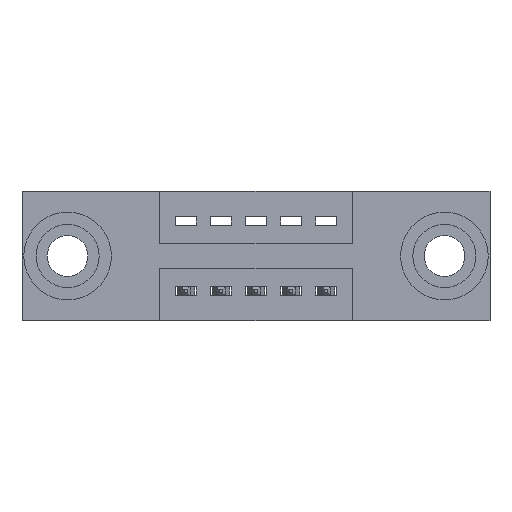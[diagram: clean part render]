
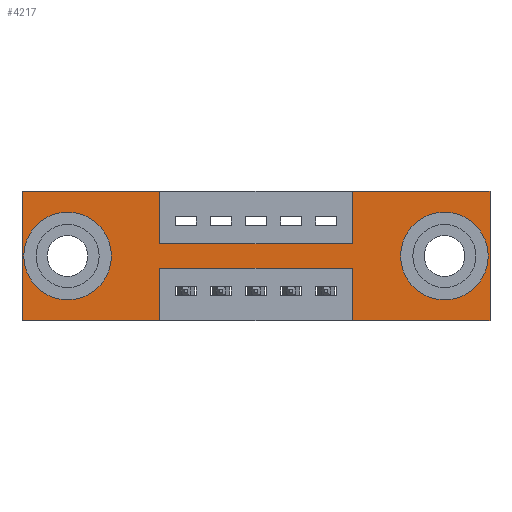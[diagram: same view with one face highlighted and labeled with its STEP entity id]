
A CAD part, front view. The second image highlights one B-rep face of the part: STEP entity #4217.
In plain terms, the highlighted planar face has unit normal (0, -1, 0).
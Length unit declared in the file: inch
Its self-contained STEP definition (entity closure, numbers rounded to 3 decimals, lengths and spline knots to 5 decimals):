
#105 = EDGE_LOOP ( 'NONE', ( #6831, #120 ) ) ;
#120 = ORIENTED_EDGE ( 'NONE', *, *, #6569, .T. ) ;
#125 = VERTEX_POINT ( 'NONE', #3889 ) ;
#225 = VECTOR ( 'NONE', #2090, 39.37008 ) ;
#229 = CARTESIAN_POINT ( 'NONE',  ( 1.335, 0., -0.37 ) ) ;
#293 = CARTESIAN_POINT ( 'NONE',  ( 0.9425, 0., -0.22 ) ) ;
#619 = CARTESIAN_POINT ( 'NONE',  ( 0.3925, 0., -0.22 ) ) ;
#776 = VERTEX_POINT ( 'NONE', #5453 ) ;
#825 = CARTESIAN_POINT ( 'NONE',  ( 1.205, 0., -0.107 ) ) ;
#836 = VERTEX_POINT ( 'NONE', #619 ) ;
#940 = CARTESIAN_POINT ( 'NONE',  ( 1.205, 0., -0.263 ) ) ;
#979 = CARTESIAN_POINT ( 'NONE',  ( 0.9425, 0., 0. ) ) ;
#1103 = VERTEX_POINT ( 'NONE', #940 ) ;
#1219 = EDGE_LOOP ( 'NONE', ( #5850, #8326 ) ) ;
#1269 = ORIENTED_EDGE ( 'NONE', *, *, #9436, .F. ) ;
#1296 = DIRECTION ( 'NONE',  ( 0., 0., 1. ) ) ;
#1366 = DIRECTION ( 'NONE',  ( 1., 0., 0. ) ) ;
#1385 = CARTESIAN_POINT ( 'NONE',  ( 0.3925, 0., -0.37 ) ) ;
#1559 = DIRECTION ( 'NONE',  ( 0., 0., -1. ) ) ;
#1603 = VECTOR ( 'NONE', #8986, 39.37008 ) ;
#1607 = VERTEX_POINT ( 'NONE', #6521 ) ;
#1641 = CARTESIAN_POINT ( 'NONE',  ( 1.335, 0., 0. ) ) ;
#1731 = VECTOR ( 'NONE', #6525, 39.37008 ) ;
#1736 = CARTESIAN_POINT ( 'NONE',  ( 0.13, 0., -0.185 ) ) ;
#1883 = LINE ( 'NONE', #6690, #5174 ) ;
#1886 = EDGE_CURVE ( 'NONE', #6975, #7728, #7655, .T. ) ;
#1965 = CARTESIAN_POINT ( 'NONE',  ( 0.3925, 0., -0.15 ) ) ;
#2052 = ORIENTED_EDGE ( 'NONE', *, *, #8198, .F. ) ;
#2064 = VERTEX_POINT ( 'NONE', #6834 ) ;
#2090 = DIRECTION ( 'NONE',  ( -1., 0., 0. ) ) ;
#2129 = VECTOR ( 'NONE', #8199, 39.37008 ) ;
#2151 = CARTESIAN_POINT ( 'NONE',  ( 0.13, 0., -0.107 ) ) ;
#2332 = DIRECTION ( 'NONE',  ( -1., 0., 0. ) ) ;
#2382 = EDGE_CURVE ( 'NONE', #7166, #836, #9350, .T. ) ;
#2756 = CIRCLE ( 'NONE', #5691, 0.078 ) ;
#2778 = VERTEX_POINT ( 'NONE', #7243 ) ;
#2874 = VECTOR ( 'NONE', #7287, 39.37008 ) ;
#2988 = ORIENTED_EDGE ( 'NONE', *, *, #9241, .F. ) ;
#3057 = DIRECTION ( 'NONE',  ( 0., 0., -1. ) ) ;
#3080 = EDGE_CURVE ( 'NONE', #7728, #4168, #4120, .T. ) ;
#3214 = DIRECTION ( 'NONE',  ( 1., 0., 0. ) ) ;
#3294 = LINE ( 'NONE', #8332, #4746 ) ;
#3483 = CARTESIAN_POINT ( 'NONE',  ( 0.13, 0., -0.185 ) ) ;
#3536 = EDGE_CURVE ( 'NONE', #836, #7986, #6952, .T. ) ;
#3540 = EDGE_LOOP ( 'NONE', ( #4556, #8865, #6306, #6263, #6079, #5271, #8102, #2988, #2052, #1269, #8885, #6864 ) ) ;
#3549 = DIRECTION ( 'NONE',  ( 0., 0., 1. ) ) ;
#3660 = FACE_BOUND ( 'NONE', #1219, .T. ) ;
#3715 = AXIS2_PLACEMENT_3D ( 'NONE', #5158, #4472, #3057 ) ;
#3751 = CARTESIAN_POINT ( 'NONE',  ( 1.205, 0., -0.185 ) ) ;
#3779 = CARTESIAN_POINT ( 'NONE',  ( 1.205, 0., -0.185 ) ) ;
#3889 = CARTESIAN_POINT ( 'NONE',  ( 0.13, 0., -0.263 ) ) ;
#3895 = VERTEX_POINT ( 'NONE', #1965 ) ;
#3916 = EDGE_CURVE ( 'NONE', #8758, #125, #2756, .T. ) ;
#4033 = LINE ( 'NONE', #4242, #1731 ) ;
#4120 = LINE ( 'NONE', #1641, #1603 ) ;
#4168 = VERTEX_POINT ( 'NONE', #229 ) ;
#4217 = ADVANCED_FACE ( 'NONE', ( #3660, #6373, #7477 ), #6607, .T. ) ;
#4242 = CARTESIAN_POINT ( 'NONE',  ( 0.3925, 0., 0. ) ) ;
#4390 = CARTESIAN_POINT ( 'NONE',  ( 1.335, 0., 0. ) ) ;
#4472 = DIRECTION ( 'NONE',  ( 0., -1., 0. ) ) ;
#4489 = DIRECTION ( 'NONE',  ( 0., 0., -1. ) ) ;
#4556 = ORIENTED_EDGE ( 'NONE', *, *, #3536, .F. ) ;
#4608 = CARTESIAN_POINT ( 'NONE',  ( 0.3925, 0., 0. ) ) ;
#4684 = DIRECTION ( 'NONE',  ( 0., 0., 1. ) ) ;
#4746 = VECTOR ( 'NONE', #3214, 39.37008 ) ;
#4811 = CARTESIAN_POINT ( 'NONE',  ( 0., 0., 0. ) ) ;
#4945 = EDGE_CURVE ( 'NONE', #1103, #7523, #7583, .T. ) ;
#4953 = EDGE_CURVE ( 'NONE', #7523, #1103, #6022, .T. ) ;
#4983 = CARTESIAN_POINT ( 'NONE',  ( 0.3925, 0., -0.15 ) ) ;
#5158 = CARTESIAN_POINT ( 'NONE',  ( 0., 0., -0.37 ) ) ;
#5174 = VECTOR ( 'NONE', #2332, 39.37008 ) ;
#5271 = ORIENTED_EDGE ( 'NONE', *, *, #1886, .F. ) ;
#5296 = CIRCLE ( 'NONE', #7233, 0.078 ) ;
#5425 = VERTEX_POINT ( 'NONE', #4608 ) ;
#5453 = CARTESIAN_POINT ( 'NONE',  ( 0.9425, 0., -0.37 ) ) ;
#5495 = VECTOR ( 'NONE', #9234, 39.37008 ) ;
#5604 = CARTESIAN_POINT ( 'NONE',  ( 0.3925, 0., -0.37 ) ) ;
#5643 = CARTESIAN_POINT ( 'NONE',  ( 0., 0., -0.37 ) ) ;
#5691 = AXIS2_PLACEMENT_3D ( 'NONE', #3483, #9279, #3549 ) ;
#5850 = ORIENTED_EDGE ( 'NONE', *, *, #4953, .T. ) ;
#6022 = CIRCLE ( 'NONE', #7044, 0.078 ) ;
#6079 = ORIENTED_EDGE ( 'NONE', *, *, #3080, .F. ) ;
#6263 = ORIENTED_EDGE ( 'NONE', *, *, #8313, .F. ) ;
#6306 = ORIENTED_EDGE ( 'NONE', *, *, #7602, .F. ) ;
#6373 = FACE_BOUND ( 'NONE', #105, .T. ) ;
#6407 = VECTOR ( 'NONE', #8268, 39.37008 ) ;
#6513 = EDGE_CURVE ( 'NONE', #2064, #2778, #8942, .T. ) ;
#6521 = CARTESIAN_POINT ( 'NONE',  ( 0.9425, 0., -0.15 ) ) ;
#6525 = DIRECTION ( 'NONE',  ( 0., 0., -1. ) ) ;
#6569 = EDGE_CURVE ( 'NONE', #125, #8758, #5296, .T. ) ;
#6607 = PLANE ( 'NONE',  #3715 ) ;
#6690 = CARTESIAN_POINT ( 'NONE',  ( 0., 0., -0.37 ) ) ;
#6812 = LINE ( 'NONE', #979, #2129 ) ;
#6831 = ORIENTED_EDGE ( 'NONE', *, *, #3916, .T. ) ;
#6834 = CARTESIAN_POINT ( 'NONE',  ( 0., 0., -0.37 ) ) ;
#6864 = ORIENTED_EDGE ( 'NONE', *, *, #8636, .F. ) ;
#6952 = LINE ( 'NONE', #1385, #2874 ) ;
#6975 = VERTEX_POINT ( 'NONE', #8677 ) ;
#7039 = LINE ( 'NONE', #5643, #225 ) ;
#7044 = AXIS2_PLACEMENT_3D ( 'NONE', #3779, #8836, #4489 ) ;
#7053 = CARTESIAN_POINT ( 'NONE',  ( 0.9425, 0., -0.37 ) ) ;
#7166 = VERTEX_POINT ( 'NONE', #293 ) ;
#7213 = VECTOR ( 'NONE', #1296, 39.37008 ) ;
#7229 = VECTOR ( 'NONE', #8879, 39.37008 ) ;
#7233 = AXIS2_PLACEMENT_3D ( 'NONE', #1736, #8321, #4684 ) ;
#7243 = CARTESIAN_POINT ( 'NONE',  ( 0., 0., 0. ) ) ;
#7287 = DIRECTION ( 'NONE',  ( 0., 0., -1. ) ) ;
#7477 = FACE_OUTER_BOUND ( 'NONE', #3540, .T. ) ;
#7490 = CARTESIAN_POINT ( 'NONE',  ( 0.3925, 0., -0.22 ) ) ;
#7523 = VERTEX_POINT ( 'NONE', #825 ) ;
#7579 = VECTOR ( 'NONE', #1366, 39.37008 ) ;
#7583 = CIRCLE ( 'NONE', #8872, 0.078 ) ;
#7602 = EDGE_CURVE ( 'NONE', #776, #7166, #8131, .T. ) ;
#7655 = LINE ( 'NONE', #4811, #5495 ) ;
#7728 = VERTEX_POINT ( 'NONE', #4390 ) ;
#7986 = VERTEX_POINT ( 'NONE', #5604 ) ;
#8102 = ORIENTED_EDGE ( 'NONE', *, *, #9372, .F. ) ;
#8109 = CARTESIAN_POINT ( 'NONE',  ( 0., 0., 0. ) ) ;
#8131 = LINE ( 'NONE', #7053, #7213 ) ;
#8198 = EDGE_CURVE ( 'NONE', #5425, #3895, #4033, .T. ) ;
#8199 = DIRECTION ( 'NONE',  ( 0., 0., 1. ) ) ;
#8268 = DIRECTION ( 'NONE',  ( -1., 0., 0. ) ) ;
#8313 = EDGE_CURVE ( 'NONE', #4168, #776, #1883, .T. ) ;
#8321 = DIRECTION ( 'NONE',  ( 0., 1., 0. ) ) ;
#8326 = ORIENTED_EDGE ( 'NONE', *, *, #4945, .T. ) ;
#8332 = CARTESIAN_POINT ( 'NONE',  ( 0., 0., 0. ) ) ;
#8636 = EDGE_CURVE ( 'NONE', #7986, #2064, #7039, .T. ) ;
#8677 = CARTESIAN_POINT ( 'NONE',  ( 0.9425, 0., 0. ) ) ;
#8758 = VERTEX_POINT ( 'NONE', #2151 ) ;
#8774 = DIRECTION ( 'NONE',  ( 0., 1., 0. ) ) ;
#8836 = DIRECTION ( 'NONE',  ( 0., 1., 0. ) ) ;
#8865 = ORIENTED_EDGE ( 'NONE', *, *, #2382, .F. ) ;
#8872 = AXIS2_PLACEMENT_3D ( 'NONE', #3751, #8774, #1559 ) ;
#8879 = DIRECTION ( 'NONE',  ( 0., 0., 1. ) ) ;
#8885 = ORIENTED_EDGE ( 'NONE', *, *, #6513, .F. ) ;
#8942 = LINE ( 'NONE', #8109, #7229 ) ;
#8949 = LINE ( 'NONE', #4983, #7579 ) ;
#8986 = DIRECTION ( 'NONE',  ( 0., 0., -1. ) ) ;
#9234 = DIRECTION ( 'NONE',  ( 1., 0., 0. ) ) ;
#9241 = EDGE_CURVE ( 'NONE', #3895, #1607, #8949, .T. ) ;
#9279 = DIRECTION ( 'NONE',  ( 0., 1., 0. ) ) ;
#9350 = LINE ( 'NONE', #7490, #6407 ) ;
#9372 = EDGE_CURVE ( 'NONE', #1607, #6975, #6812, .T. ) ;
#9436 = EDGE_CURVE ( 'NONE', #2778, #5425, #3294, .T. ) ;
